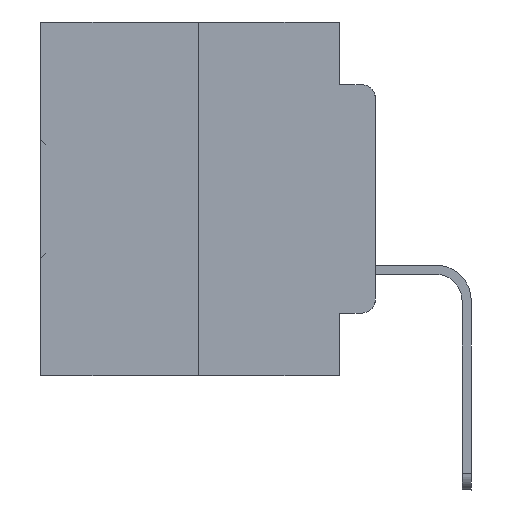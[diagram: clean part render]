
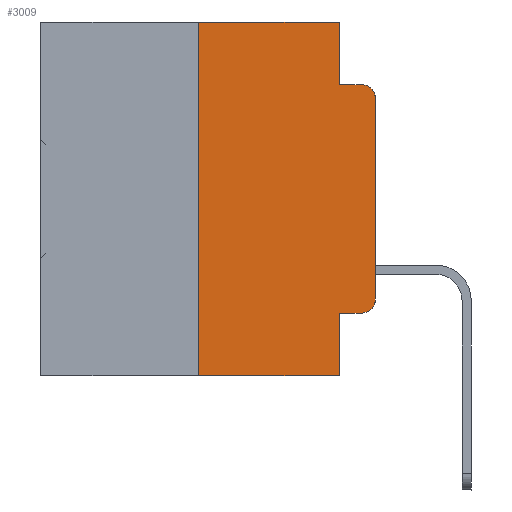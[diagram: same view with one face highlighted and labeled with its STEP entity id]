
A CAD part, left-side view. The second image highlights one B-rep face of the part: STEP entity #3009.
In plain terms, the highlighted planar face has unit normal (-1, 0, 0).
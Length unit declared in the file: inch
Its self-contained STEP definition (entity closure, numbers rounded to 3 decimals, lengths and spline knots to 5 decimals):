
#56 = CARTESIAN_POINT ( 'NONE',  ( 0., 0.473, -0.5 ) ) ;
#192 = ORIENTED_EDGE ( 'NONE', *, *, #10907, .T. ) ;
#196 = CARTESIAN_POINT ( 'NONE',  ( 0., 0.02, -0.4115 ) ) ;
#208 = VECTOR ( 'NONE', #18542, 39.37008 ) ;
#347 = DIRECTION ( 'NONE',  ( 0., 0., -1. ) ) ;
#383 = ORIENTED_EDGE ( 'NONE', *, *, #30498, .F. ) ;
#718 = EDGE_CURVE ( 'NONE', #27381, #25501, #18771, .T. ) ;
#1433 = VECTOR ( 'NONE', #4724, 39.37008 ) ;
#1512 = ORIENTED_EDGE ( 'NONE', *, *, #32346, .F. ) ;
#1925 = CARTESIAN_POINT ( 'NONE',  ( 0., 0., -0.1085 ) ) ;
#2880 = ORIENTED_EDGE ( 'NONE', *, *, #10810, .T. ) ;
#3009 = ADVANCED_FACE ( 'NONE', ( #11812 ), #24907, .F. ) ;
#3122 = ORIENTED_EDGE ( 'NONE', *, *, #718, .T. ) ;
#3293 = EDGE_LOOP ( 'NONE', ( #192, #3122, #383, #1512, #30293, #31601, #12510, #3995, #2880, #16177 ) ) ;
#3355 = CARTESIAN_POINT ( 'NONE',  ( 0., 0.051, -0.4115 ) ) ;
#3995 = ORIENTED_EDGE ( 'NONE', *, *, #20187, .F. ) ;
#4041 = AXIS2_PLACEMENT_3D ( 'NONE', #7273, #22767, #30719 ) ;
#4097 = VERTEX_POINT ( 'NONE', #5604 ) ;
#4724 = DIRECTION ( 'NONE',  ( 0., 0., -1. ) ) ;
#4925 = VERTEX_POINT ( 'NONE', #196 ) ;
#5199 = CARTESIAN_POINT ( 'NONE',  ( 0., 0., -0.3915 ) ) ;
#5323 = DIRECTION ( 'NONE',  ( 0., 0., 1. ) ) ;
#5604 = CARTESIAN_POINT ( 'NONE',  ( 0., 0.25, 0. ) ) ;
#5821 = CIRCLE ( 'NONE', #10797, 0.02 ) ;
#6271 = EDGE_CURVE ( 'NONE', #4925, #18128, #5821, .T. ) ;
#6405 = CARTESIAN_POINT ( 'NONE',  ( 0., 0.051, 0. ) ) ;
#7175 = VECTOR ( 'NONE', #347, 39.37008 ) ;
#7273 = CARTESIAN_POINT ( 'NONE',  ( 0., 0.02, -0.1085 ) ) ;
#7720 = VERTEX_POINT ( 'NONE', #32947 ) ;
#7887 = CARTESIAN_POINT ( 'NONE',  ( 0., 0.051, -0.0885 ) ) ;
#8100 = LINE ( 'NONE', #12756, #1433 ) ;
#8485 = LINE ( 'NONE', #23554, #10147 ) ;
#10147 = VECTOR ( 'NONE', #31503, 39.37008 ) ;
#10797 = AXIS2_PLACEMENT_3D ( 'NONE', #27591, #25155, #14403 ) ;
#10809 = CARTESIAN_POINT ( 'NONE',  ( 0., 0.473, 0. ) ) ;
#10810 = EDGE_CURVE ( 'NONE', #21160, #4925, #18095, .T. ) ;
#10907 = EDGE_CURVE ( 'NONE', #18128, #27381, #15587, .T. ) ;
#11781 = VERTEX_POINT ( 'NONE', #29932 ) ;
#11812 = FACE_OUTER_BOUND ( 'NONE', #3293, .T. ) ;
#12187 = LINE ( 'NONE', #10809, #32431 ) ;
#12290 = LINE ( 'NONE', #7887, #208 ) ;
#12510 = ORIENTED_EDGE ( 'NONE', *, *, #16647, .T. ) ;
#12756 = CARTESIAN_POINT ( 'NONE',  ( 0., 0.051, 0. ) ) ;
#12774 = VERTEX_POINT ( 'NONE', #18234 ) ;
#14299 = EDGE_CURVE ( 'NONE', #11781, #4097, #8485, .T. ) ;
#14403 = DIRECTION ( 'NONE',  ( 0., 0., -1. ) ) ;
#15587 = LINE ( 'NONE', #23630, #23867 ) ;
#16006 = VECTOR ( 'NONE', #28381, 39.37008 ) ;
#16177 = ORIENTED_EDGE ( 'NONE', *, *, #6271, .T. ) ;
#16647 = EDGE_CURVE ( 'NONE', #11781, #12774, #21192, .T. ) ;
#16662 = CARTESIAN_POINT ( 'NONE',  ( 0., 0.02, -0.0885 ) ) ;
#18095 = LINE ( 'NONE', #23181, #16006 ) ;
#18128 = VERTEX_POINT ( 'NONE', #5199 ) ;
#18234 = CARTESIAN_POINT ( 'NONE',  ( 0., 0.051, -0.5 ) ) ;
#18542 = DIRECTION ( 'NONE',  ( 0., -1., 0. ) ) ;
#18629 = DIRECTION ( 'NONE',  ( 0., -1., 0. ) ) ;
#18771 = CIRCLE ( 'NONE', #4041, 0.02 ) ;
#20187 = EDGE_CURVE ( 'NONE', #21160, #12774, #33227, .T. ) ;
#21160 = VERTEX_POINT ( 'NONE', #3355 ) ;
#21192 = LINE ( 'NONE', #56, #31122 ) ;
#21316 = DIRECTION ( 'NONE',  ( 0., -1., 0. ) ) ;
#22767 = DIRECTION ( 'NONE',  ( -1., 0., 0. ) ) ;
#23181 = CARTESIAN_POINT ( 'NONE',  ( 0., 0.051, -0.4115 ) ) ;
#23554 = CARTESIAN_POINT ( 'NONE',  ( 0., 0.25, 0. ) ) ;
#23630 = CARTESIAN_POINT ( 'NONE',  ( 0., 0., 0. ) ) ;
#23822 = AXIS2_PLACEMENT_3D ( 'NONE', #32755, #27907, #32987 ) ;
#23867 = VECTOR ( 'NONE', #5323, 39.37008 ) ;
#24907 = PLANE ( 'NONE',  #23822 ) ;
#25155 = DIRECTION ( 'NONE',  ( -1., 0., 0. ) ) ;
#25501 = VERTEX_POINT ( 'NONE', #16662 ) ;
#27381 = VERTEX_POINT ( 'NONE', #1925 ) ;
#27591 = CARTESIAN_POINT ( 'NONE',  ( 0., 0.02, -0.3915 ) ) ;
#27907 = DIRECTION ( 'NONE',  ( 1., 0., 0. ) ) ;
#28381 = DIRECTION ( 'NONE',  ( 0., -1., 0. ) ) ;
#29402 = CARTESIAN_POINT ( 'NONE',  ( 0., 0.051, 0. ) ) ;
#29932 = CARTESIAN_POINT ( 'NONE',  ( 0., 0.25, -0.5 ) ) ;
#30293 = ORIENTED_EDGE ( 'NONE', *, *, #31893, .F. ) ;
#30338 = VERTEX_POINT ( 'NONE', #6405 ) ;
#30498 = EDGE_CURVE ( 'NONE', #7720, #25501, #12290, .T. ) ;
#30719 = DIRECTION ( 'NONE',  ( 0., 0., -1. ) ) ;
#31122 = VECTOR ( 'NONE', #18629, 39.37008 ) ;
#31503 = DIRECTION ( 'NONE',  ( 0., 0., 1. ) ) ;
#31601 = ORIENTED_EDGE ( 'NONE', *, *, #14299, .F. ) ;
#31893 = EDGE_CURVE ( 'NONE', #4097, #30338, #12187, .T. ) ;
#32346 = EDGE_CURVE ( 'NONE', #30338, #7720, #8100, .T. ) ;
#32431 = VECTOR ( 'NONE', #21316, 39.37008 ) ;
#32755 = CARTESIAN_POINT ( 'NONE',  ( 0., 0.473, 0. ) ) ;
#32947 = CARTESIAN_POINT ( 'NONE',  ( 0., 0.051, -0.0885 ) ) ;
#32987 = DIRECTION ( 'NONE',  ( 0., 0., -1. ) ) ;
#33227 = LINE ( 'NONE', #29402, #7175 ) ;
